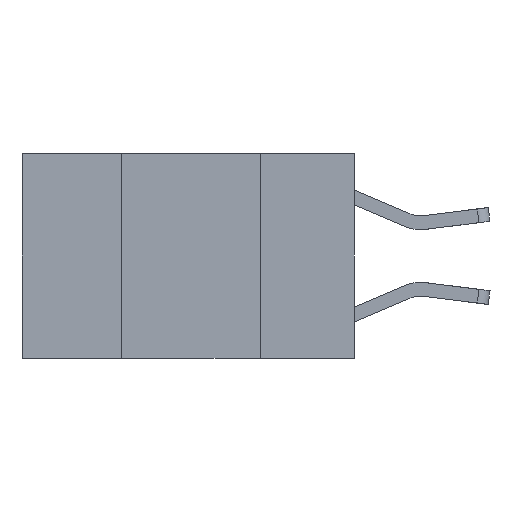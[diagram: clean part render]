
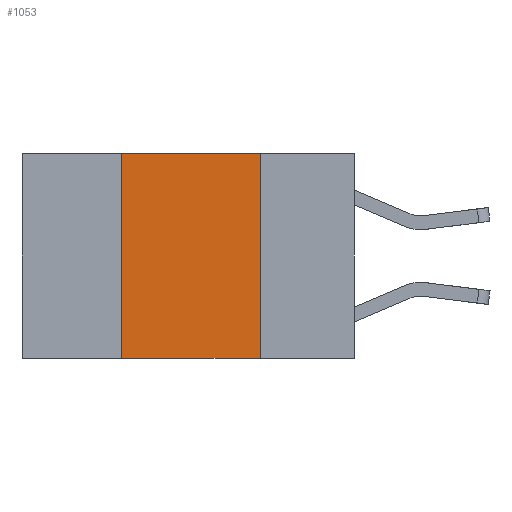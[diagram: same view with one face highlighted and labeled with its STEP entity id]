
A CAD part, left-side view. The second image highlights one B-rep face of the part: STEP entity #1053.
In plain terms, the highlighted planar face has unit normal (-1, 0, 0).
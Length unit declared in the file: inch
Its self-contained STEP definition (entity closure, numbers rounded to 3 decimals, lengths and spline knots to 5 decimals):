
#49 = EDGE_CURVE ( 'NONE', #810, #2822, #4726, .T. ) ;
#448 = DIRECTION ( 'NONE',  ( 0., -1., 0. ) ) ;
#810 = VERTEX_POINT ( 'NONE', #5805 ) ;
#1053 = ADVANCED_FACE ( 'NONE', ( #9103 ), #7416, .F. ) ;
#1119 = VECTOR ( 'NONE', #7899, 39.37008 ) ;
#1675 = ORIENTED_EDGE ( 'NONE', *, *, #49, .F. ) ;
#1998 = ORIENTED_EDGE ( 'NONE', *, *, #7211, .F. ) ;
#2311 = VECTOR ( 'NONE', #7466, 39.37008 ) ;
#2822 = VERTEX_POINT ( 'NONE', #8179 ) ;
#2853 = VERTEX_POINT ( 'NONE', #6255 ) ;
#3481 = LINE ( 'NONE', #7017, #1119 ) ;
#3482 = CARTESIAN_POINT ( 'NONE',  ( 0., 0.6, 0. ) ) ;
#3611 = LINE ( 'NONE', #9784, #9935 ) ;
#3921 = CARTESIAN_POINT ( 'NONE',  ( 0., 0.17, 0. ) ) ;
#4012 = LINE ( 'NONE', #8076, #10316 ) ;
#4726 = LINE ( 'NONE', #3921, #2311 ) ;
#4860 = ORIENTED_EDGE ( 'NONE', *, *, #6203, .F. ) ;
#5624 = VERTEX_POINT ( 'NONE', #5812 ) ;
#5805 = CARTESIAN_POINT ( 'NONE',  ( 0., 0.17, 0. ) ) ;
#5812 = CARTESIAN_POINT ( 'NONE',  ( 0., 0.42, -0.37 ) ) ;
#6203 = EDGE_CURVE ( 'NONE', #5624, #2853, #4012, .T. ) ;
#6255 = CARTESIAN_POINT ( 'NONE',  ( 0., 0.42, 0. ) ) ;
#6458 = EDGE_LOOP ( 'NONE', ( #1675, #1998, #4860, #8728 ) ) ;
#7017 = CARTESIAN_POINT ( 'NONE',  ( 0., 0.6, -0.37 ) ) ;
#7211 = EDGE_CURVE ( 'NONE', #2853, #810, #3611, .T. ) ;
#7416 = PLANE ( 'NONE',  #10801 ) ;
#7466 = DIRECTION ( 'NONE',  ( 0., 0., -1. ) ) ;
#7770 = EDGE_CURVE ( 'NONE', #5624, #2822, #3481, .T. ) ;
#7899 = DIRECTION ( 'NONE',  ( 0., -1., 0. ) ) ;
#8076 = CARTESIAN_POINT ( 'NONE',  ( 0., 0.42, 0. ) ) ;
#8132 = DIRECTION ( 'NONE',  ( 1., 0., 0. ) ) ;
#8179 = CARTESIAN_POINT ( 'NONE',  ( 0., 0.17, -0.37 ) ) ;
#8207 = DIRECTION ( 'NONE',  ( 0., 0., -1. ) ) ;
#8728 = ORIENTED_EDGE ( 'NONE', *, *, #7770, .T. ) ;
#8885 = DIRECTION ( 'NONE',  ( 0., 0., 1. ) ) ;
#9103 = FACE_OUTER_BOUND ( 'NONE', #6458, .T. ) ;
#9784 = CARTESIAN_POINT ( 'NONE',  ( 0., 0.6, 0. ) ) ;
#9935 = VECTOR ( 'NONE', #448, 39.37008 ) ;
#10316 = VECTOR ( 'NONE', #8885, 39.37008 ) ;
#10801 = AXIS2_PLACEMENT_3D ( 'NONE', #3482, #8132, #8207 ) ;
